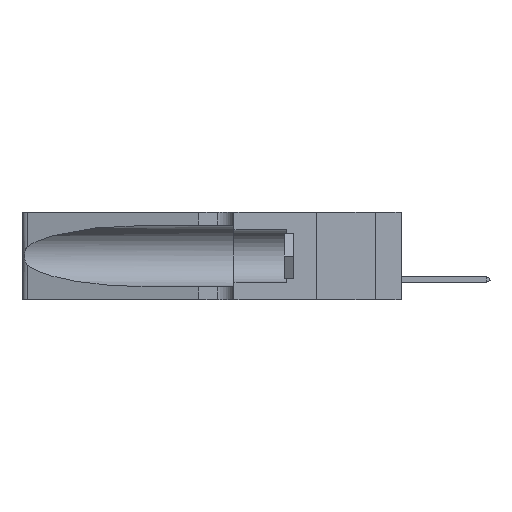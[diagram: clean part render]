
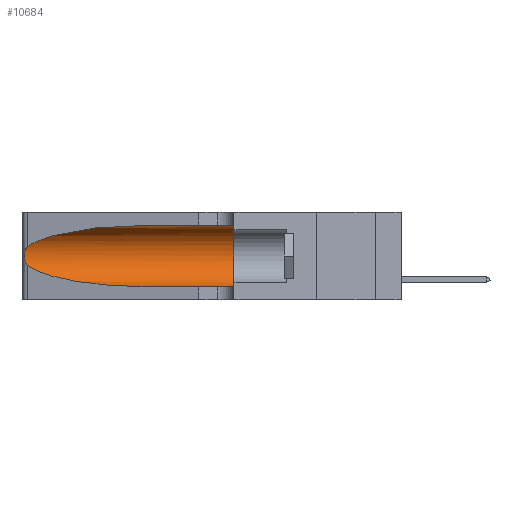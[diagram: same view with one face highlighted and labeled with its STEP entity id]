
A CAD part, left-side view. The second image highlights one B-rep face of the part: STEP entity #10684.
In plain terms, the highlighted cylindrical face has radius 3.308 mm (diameter 6.617 mm), a partial arc.
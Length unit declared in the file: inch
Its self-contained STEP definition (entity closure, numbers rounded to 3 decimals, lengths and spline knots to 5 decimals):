
#192 = B_SPLINE_CURVE_WITH_KNOTS ( 'NONE', 3,
 ( #17630, #4469, #1044, #3170, #23770, #3327, #1528, #5279, #16718, #21377, #17101, #13995, #23240, #19032 ),
 .UNSPECIFIED., .F., .F.,
 ( 4, 2, 2, 2, 2, 2, 4 ),
 ( 0., 0.00027, 0.00053, 0.00107, 0.0016, 0.00187, 0.00214 ),
 .UNSPECIFIED. ) ;
#343 = DIRECTION ( 'NONE',  ( 0., 0., 1. ) ) ;
#717 = CARTESIAN_POINT ( 'NONE',  ( 0.1305, 1.61858, 0.31525 ) ) ;
#1044 = CARTESIAN_POINT ( 'NONE',  ( 0.25639, 1.23184, 0.21858 ) ) ;
#1067 = EDGE_CURVE ( 'NONE', #8020, #17763, #17150, .T. ) ;
#1089 = DIRECTION ( 'NONE',  ( 0., -1., 0. ) ) ;
#1528 = CARTESIAN_POINT ( 'NONE',  ( 0.26075, 1.23896, 0.19203 ) ) ;
#1716 = ORIENTED_EDGE ( 'NONE', *, *, #17354, .F. ) ;
#2478 = CARTESIAN_POINT ( 'NONE',  ( 0.18966, 0.96281, 0.31525 ) ) ;
#3004 =( BOUNDED_CURVE ( )  B_SPLINE_CURVE ( 3, ( #17269, #2478, #11714, #6451 ),
 .UNSPECIFIED., .F., .F. ) 
 B_SPLINE_CURVE_WITH_KNOTS ( ( 4, 4 ),
 ( 1.5708, 2.84003 ),
 .UNSPECIFIED. ) 
 CURVE ( )  GEOMETRIC_REPRESENTATION_ITEM ( )  RATIONAL_B_SPLINE_CURVE ( ( 1., 0.87, 0.87, 1. ) ) 
 REPRESENTATION_ITEM ( '' )  );
#3170 = CARTESIAN_POINT ( 'NONE',  ( 0.25787, 1.23484, 0.2124 ) ) ;
#3327 = CARTESIAN_POINT ( 'NONE',  ( 0.26018, 1.23835, 0.19895 ) ) ;
#3606 = CARTESIAN_POINT ( 'NONE',  ( 0.25487, 1.22718, 0.14631 ) ) ;
#4469 = CARTESIAN_POINT ( 'NONE',  ( 0.25555, 1.22994, 0.2215 ) ) ;
#4555 = AXIS2_PLACEMENT_3D ( 'NONE', #20103, #12691, #7333 ) ;
#4848 = VERTEX_POINT ( 'NONE', #14809 ) ;
#5023 = FACE_OUTER_BOUND ( 'NONE', #9705, .T. ) ;
#5191 = CARTESIAN_POINT ( 'NONE',  ( 0.1305, 0.35, 0.05475 ) ) ;
#5279 = CARTESIAN_POINT ( 'NONE',  ( 0.26075, 1.23896, 0.178 ) ) ;
#6451 = CARTESIAN_POINT ( 'NONE',  ( 0.25487, 1.22718, 0.22369 ) ) ;
#6736 = CARTESIAN_POINT ( 'NONE',  ( 0.18966, 0.96281, 0.05475 ) ) ;
#7333 = DIRECTION ( 'NONE',  ( 0., 0., -1. ) ) ;
#7610 = CYLINDRICAL_SURFACE ( 'NONE', #4555, 0.13025 ) ;
#7803 = CARTESIAN_POINT ( 'NONE',  ( 0.25487, 1.22718, 0.22369 ) ) ;
#8020 = VERTEX_POINT ( 'NONE', #3606 ) ;
#8094 = LINE ( 'NONE', #717, #22356 ) ;
#9201 = ORIENTED_EDGE ( 'NONE', *, *, #23609, .F. ) ;
#9595 = VECTOR ( 'NONE', #1089, 39.37008 ) ;
#9705 = EDGE_LOOP ( 'NONE', ( #20975, #21851, #18842, #16557, #9201, #1716 ) ) ;
#10236 = EDGE_CURVE ( 'NONE', #4848, #19562, #3004, .T. ) ;
#10249 = VERTEX_POINT ( 'NONE', #16104 ) ;
#10684 = ADVANCED_FACE ( 'NONE', ( #5023 ), #7610, .F. ) ;
#11285 = EDGE_CURVE ( 'NONE', #17763, #21900, #22432, .T. ) ;
#11431 = DIRECTION ( 'NONE',  ( 0., 1., 0. ) ) ;
#11714 = CARTESIAN_POINT ( 'NONE',  ( 0.2373, 1.15595, 0.28018 ) ) ;
#12691 = DIRECTION ( 'NONE',  ( 0., -1., 0. ) ) ;
#13995 = CARTESIAN_POINT ( 'NONE',  ( 0.25639, 1.23186, 0.15144 ) ) ;
#14809 = CARTESIAN_POINT ( 'NONE',  ( 0.1305, 0.72297, 0.31525 ) ) ;
#15085 = AXIS2_PLACEMENT_3D ( 'NONE', #22566, #11431, #343 ) ;
#16012 = EDGE_CURVE ( 'NONE', #19562, #8020, #192, .T. ) ;
#16104 = CARTESIAN_POINT ( 'NONE',  ( 0.1305, 0.35, 0.31525 ) ) ;
#16133 = DIRECTION ( 'NONE',  ( 0., -1., 0. ) ) ;
#16557 = ORIENTED_EDGE ( 'NONE', *, *, #11285, .T. ) ;
#16618 = CIRCLE ( 'NONE', #15085, 0.13025 ) ;
#16718 = CARTESIAN_POINT ( 'NONE',  ( 0.26017, 1.23833, 0.17102 ) ) ;
#17101 = CARTESIAN_POINT ( 'NONE',  ( 0.25789, 1.23486, 0.15765 ) ) ;
#17150 =( BOUNDED_CURVE ( )  B_SPLINE_CURVE ( 3, ( #23463, #21443, #6736, #23548 ),
 .UNSPECIFIED., .F., .T. ) 
 B_SPLINE_CURVE_WITH_KNOTS ( ( 4, 4 ),
 ( 3.44316, 4.71239 ),
 .UNSPECIFIED. ) 
 CURVE ( )  GEOMETRIC_REPRESENTATION_ITEM ( )  RATIONAL_B_SPLINE_CURVE ( ( 1., 0.87, 0.87, 1. ) ) 
 REPRESENTATION_ITEM ( '' )  );
#17269 = CARTESIAN_POINT ( 'NONE',  ( 0.1305, 0.72297, 0.31525 ) ) ;
#17354 = EDGE_CURVE ( 'NONE', #4848, #10249, #8094, .T. ) ;
#17630 = CARTESIAN_POINT ( 'NONE',  ( 0.25487, 1.22718, 0.22369 ) ) ;
#17763 = VERTEX_POINT ( 'NONE', #21348 ) ;
#18842 = ORIENTED_EDGE ( 'NONE', *, *, #1067, .T. ) ;
#19032 = CARTESIAN_POINT ( 'NONE',  ( 0.25487, 1.22718, 0.14631 ) ) ;
#19562 = VERTEX_POINT ( 'NONE', #7803 ) ;
#20103 = CARTESIAN_POINT ( 'NONE',  ( 0.1305, 1.61858, 0.185 ) ) ;
#20975 = ORIENTED_EDGE ( 'NONE', *, *, #10236, .T. ) ;
#21348 = CARTESIAN_POINT ( 'NONE',  ( 0.1305, 0.72297, 0.05475 ) ) ;
#21377 = CARTESIAN_POINT ( 'NONE',  ( 0.25856, 1.23593, 0.16098 ) ) ;
#21443 = CARTESIAN_POINT ( 'NONE',  ( 0.2373, 1.15595, 0.08982 ) ) ;
#21851 = ORIENTED_EDGE ( 'NONE', *, *, #16012, .T. ) ;
#21900 = VERTEX_POINT ( 'NONE', #5191 ) ;
#22356 = VECTOR ( 'NONE', #16133, 39.37008 ) ;
#22432 = LINE ( 'NONE', #23265, #9595 ) ;
#22566 = CARTESIAN_POINT ( 'NONE',  ( 0.1305, 0.35, 0.185 ) ) ;
#23240 = CARTESIAN_POINT ( 'NONE',  ( 0.25555, 1.22993, 0.14849 ) ) ;
#23265 = CARTESIAN_POINT ( 'NONE',  ( 0.1305, 1.61858, 0.05475 ) ) ;
#23463 = CARTESIAN_POINT ( 'NONE',  ( 0.25487, 1.22718, 0.14631 ) ) ;
#23548 = CARTESIAN_POINT ( 'NONE',  ( 0.1305, 0.72297, 0.05475 ) ) ;
#23609 = EDGE_CURVE ( 'NONE', #10249, #21900, #16618, .T. ) ;
#23770 = CARTESIAN_POINT ( 'NONE',  ( 0.25854, 1.2359, 0.20912 ) ) ;
